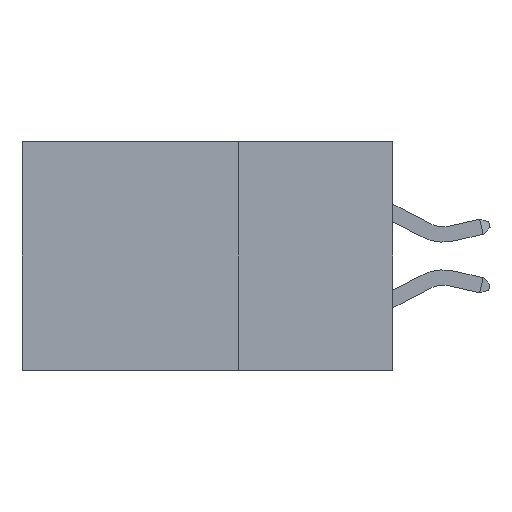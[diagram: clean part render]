
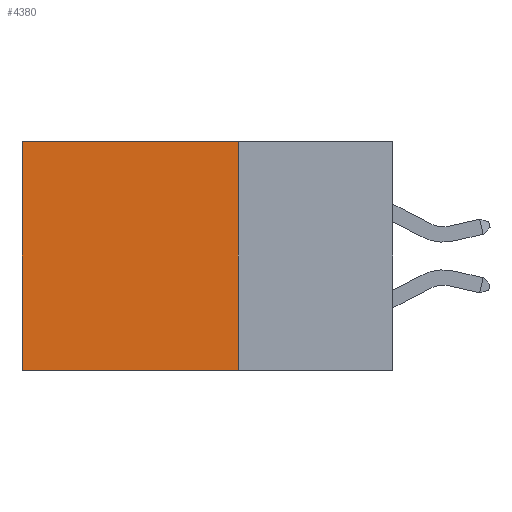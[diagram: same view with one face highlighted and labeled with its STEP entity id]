
A CAD part, left-side view. The second image highlights one B-rep face of the part: STEP entity #4380.
In plain terms, the highlighted planar face has unit normal (-1, 0, 0).
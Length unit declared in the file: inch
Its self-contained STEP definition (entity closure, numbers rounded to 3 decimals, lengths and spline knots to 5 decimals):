
#859 = DIRECTION ( 'NONE',  ( 0., 1., 0. ) ) ;
#926 = VERTEX_POINT ( 'NONE', #9908 ) ;
#973 = EDGE_CURVE ( 'NONE', #29457, #926, #31370, .T. ) ;
#1833 = PLANE ( 'NONE',  #26178 ) ;
#1908 = EDGE_CURVE ( 'NONE', #6798, #32070, #19027, .T. ) ;
#2526 = ORIENTED_EDGE ( 'NONE', *, *, #3706, .T. ) ;
#2800 = VECTOR ( 'NONE', #13780, 39.37008 ) ;
#3706 = EDGE_CURVE ( 'NONE', #32070, #926, #6729, .T. ) ;
#3871 = DIRECTION ( 'NONE',  ( 0., 0., -1. ) ) ;
#4380 = ADVANCED_FACE ( 'NONE', ( #12970 ), #1833, .F. ) ;
#4392 = DIRECTION ( 'NONE',  ( 0., 0., -1. ) ) ;
#4504 = ORIENTED_EDGE ( 'NONE', *, *, #973, .F. ) ;
#6729 = LINE ( 'NONE', #21403, #26670 ) ;
#6798 = VERTEX_POINT ( 'NONE', #30656 ) ;
#7175 = ORIENTED_EDGE ( 'NONE', *, *, #1908, .T. ) ;
#8415 = CARTESIAN_POINT ( 'NONE',  ( 0.2875, 0.25, 0. ) ) ;
#9908 = CARTESIAN_POINT ( 'NONE',  ( 0.2875, 0.6, -0.37 ) ) ;
#10011 = CARTESIAN_POINT ( 'NONE',  ( 0.2875, 0.25, -0.37 ) ) ;
#12970 = FACE_OUTER_BOUND ( 'NONE', #24467, .T. ) ;
#13780 = DIRECTION ( 'NONE',  ( 0., 0., -1. ) ) ;
#13843 = CARTESIAN_POINT ( 'NONE',  ( 0.2875, 0.25, -0.37 ) ) ;
#19027 = LINE ( 'NONE', #8415, #24851 ) ;
#19428 = DIRECTION ( 'NONE',  ( 1., 0., 0. ) ) ;
#20334 = CARTESIAN_POINT ( 'NONE',  ( 0.2875, 0.6, 0. ) ) ;
#21403 = CARTESIAN_POINT ( 'NONE',  ( 0.2875, 0.6, 0. ) ) ;
#23040 = EDGE_CURVE ( 'NONE', #6798, #29457, #30209, .T. ) ;
#24334 = CARTESIAN_POINT ( 'NONE',  ( 0.2875, 0.25, 0. ) ) ;
#24467 = EDGE_LOOP ( 'NONE', ( #2526, #4504, #28832, #7175 ) ) ;
#24788 = VECTOR ( 'NONE', #32425, 39.37008 ) ;
#24851 = VECTOR ( 'NONE', #859, 39.37008 ) ;
#26178 = AXIS2_PLACEMENT_3D ( 'NONE', #24334, #19428, #4392 ) ;
#26670 = VECTOR ( 'NONE', #3871, 39.37008 ) ;
#28832 = ORIENTED_EDGE ( 'NONE', *, *, #23040, .F. ) ;
#29457 = VERTEX_POINT ( 'NONE', #13843 ) ;
#30209 = LINE ( 'NONE', #31077, #2800 ) ;
#30656 = CARTESIAN_POINT ( 'NONE',  ( 0.2875, 0.25, 0. ) ) ;
#31077 = CARTESIAN_POINT ( 'NONE',  ( 0.2875, 0.25, 0. ) ) ;
#31370 = LINE ( 'NONE', #10011, #24788 ) ;
#32070 = VERTEX_POINT ( 'NONE', #20334 ) ;
#32425 = DIRECTION ( 'NONE',  ( 0., 1., 0. ) ) ;
